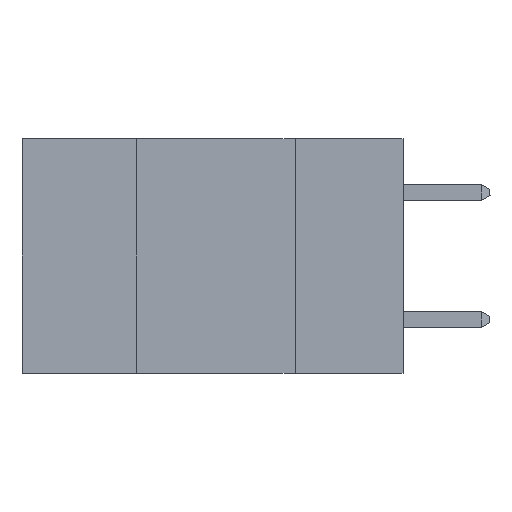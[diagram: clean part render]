
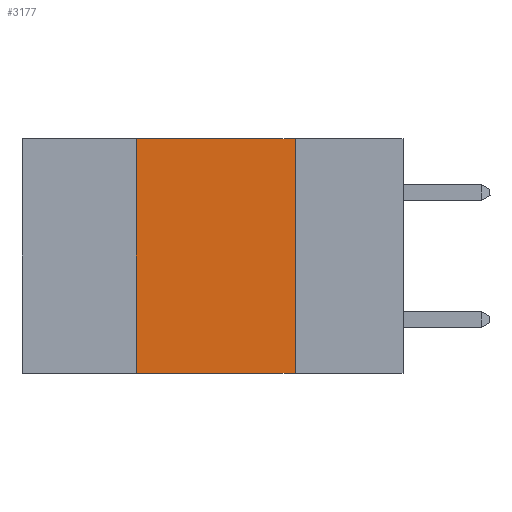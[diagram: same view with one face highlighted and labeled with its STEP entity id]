
A CAD part, left-side view. The second image highlights one B-rep face of the part: STEP entity #3177.
In plain terms, the highlighted planar face has unit normal (-1, 0, 0).
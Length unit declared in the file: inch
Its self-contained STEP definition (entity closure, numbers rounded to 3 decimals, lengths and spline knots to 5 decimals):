
#1346 = PLANE ( 'NONE',  #9266 ) ;
#1369 = CARTESIAN_POINT ( 'NONE',  ( 0., 0.6, 0. ) ) ;
#1376 = LINE ( 'NONE', #6924, #9238 ) ;
#1456 = DIRECTION ( 'NONE',  ( 0., 0., -1. ) ) ;
#1561 = CARTESIAN_POINT ( 'NONE',  ( 0., 0.6, 0. ) ) ;
#2164 = EDGE_CURVE ( 'NONE', #3869, #6180, #8480, .T. ) ;
#2278 = ORIENTED_EDGE ( 'NONE', *, *, #7317, .F. ) ;
#3177 = ADVANCED_FACE ( 'NONE', ( #8160 ), #1346, .F. ) ;
#3645 = EDGE_LOOP ( 'NONE', ( #3860, #8934, #2278, #3813 ) ) ;
#3813 = ORIENTED_EDGE ( 'NONE', *, *, #2164, .T. ) ;
#3860 = ORIENTED_EDGE ( 'NONE', *, *, #10521, .F. ) ;
#3869 = VERTEX_POINT ( 'NONE', #5669 ) ;
#4181 = DIRECTION ( 'NONE',  ( 0., -1., 0. ) ) ;
#4204 = LINE ( 'NONE', #5916, #6343 ) ;
#4269 = EDGE_CURVE ( 'NONE', #7160, #10745, #10522, .T. ) ;
#4473 = DIRECTION ( 'NONE',  ( 0., 0., 1. ) ) ;
#5151 = CARTESIAN_POINT ( 'NONE',  ( 0., 0.6, -0.37 ) ) ;
#5669 = CARTESIAN_POINT ( 'NONE',  ( 0., 0.42, -0.37 ) ) ;
#5766 = VECTOR ( 'NONE', #4181, 39.37008 ) ;
#5881 = CARTESIAN_POINT ( 'NONE',  ( 0., 0.42, 0. ) ) ;
#5916 = CARTESIAN_POINT ( 'NONE',  ( 0., 0.17, 0. ) ) ;
#6180 = VERTEX_POINT ( 'NONE', #6698 ) ;
#6343 = VECTOR ( 'NONE', #7780, 39.37008 ) ;
#6698 = CARTESIAN_POINT ( 'NONE',  ( 0., 0.17, -0.37 ) ) ;
#6924 = CARTESIAN_POINT ( 'NONE',  ( 0., 0.42, 0. ) ) ;
#7076 = DIRECTION ( 'NONE',  ( 0., -1., 0. ) ) ;
#7160 = VERTEX_POINT ( 'NONE', #5881 ) ;
#7317 = EDGE_CURVE ( 'NONE', #3869, #7160, #1376, .T. ) ;
#7780 = DIRECTION ( 'NONE',  ( 0., 0., -1. ) ) ;
#8085 = VECTOR ( 'NONE', #7076, 39.37008 ) ;
#8160 = FACE_OUTER_BOUND ( 'NONE', #3645, .T. ) ;
#8480 = LINE ( 'NONE', #5151, #5766 ) ;
#8934 = ORIENTED_EDGE ( 'NONE', *, *, #4269, .F. ) ;
#9238 = VECTOR ( 'NONE', #4473, 39.37008 ) ;
#9266 = AXIS2_PLACEMENT_3D ( 'NONE', #1561, #10561, #1456 ) ;
#10521 = EDGE_CURVE ( 'NONE', #10745, #6180, #4204, .T. ) ;
#10522 = LINE ( 'NONE', #1369, #8085 ) ;
#10561 = DIRECTION ( 'NONE',  ( 1., 0., 0. ) ) ;
#10686 = CARTESIAN_POINT ( 'NONE',  ( 0., 0.17, 0. ) ) ;
#10745 = VERTEX_POINT ( 'NONE', #10686 ) ;
